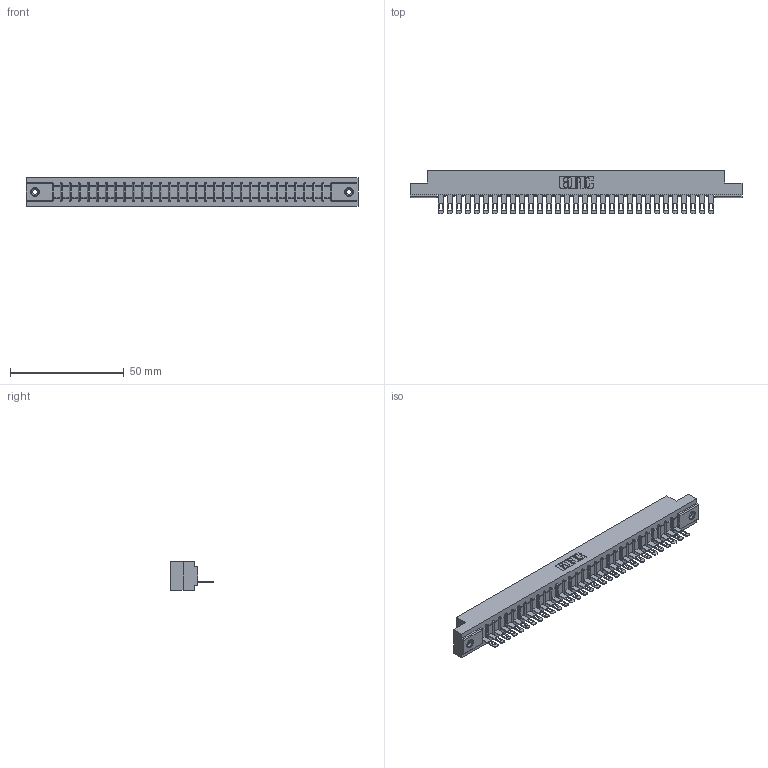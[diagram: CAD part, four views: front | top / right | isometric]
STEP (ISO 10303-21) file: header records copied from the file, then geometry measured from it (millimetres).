
FILE_DESCRIPTION (( 'STEP AP203' ), '1' );
FILE_NAME ('357-031-405-108.STEP', '2020-10-02T02:18:31', ( '' ), ( '' ), 'SwSTEP 2.0', 'SolidWorks 2020', '' );
FILE_SCHEMA (( 'CONFIG_CONTROL_DESIGN' ));
Length unit declared in the file: inch
Products named in the file (4): 307-290-001_505; 357-031-405-108; 345-250-001_345-250-003-102; 307 Part_.156 Dia Mounting Holes
Assembly tree (34 placements, depth 2):
  357-031-405-108
    307 Part_.156 Dia Mounting Holes
    307-290-001_505  x31
    345-250-001_345-250-003-102  x2
Bounding box: 145.85 x 19.18 x 12.7 mm (x, y, z)
Volume: 15113.5 mm3; surface area: 16158.5 mm2
Topology: 34 solids, 34 shells, 1946 faces, 5481 edges, 3518 vertices
Faces by surface type: plane 1218, cylinder 648, sphere 64, cone 12, torus 4
Entity records: 29091 total; most frequent: CARTESIAN_POINT 4875, ORIENTED_EDGE 4854, DIRECTION 4759, EDGE_CURVE 2427, LINE 1855, VECTOR 1855, VERTEX_POINT 1568, AXIS2_PLACEMENT_3D 1452
